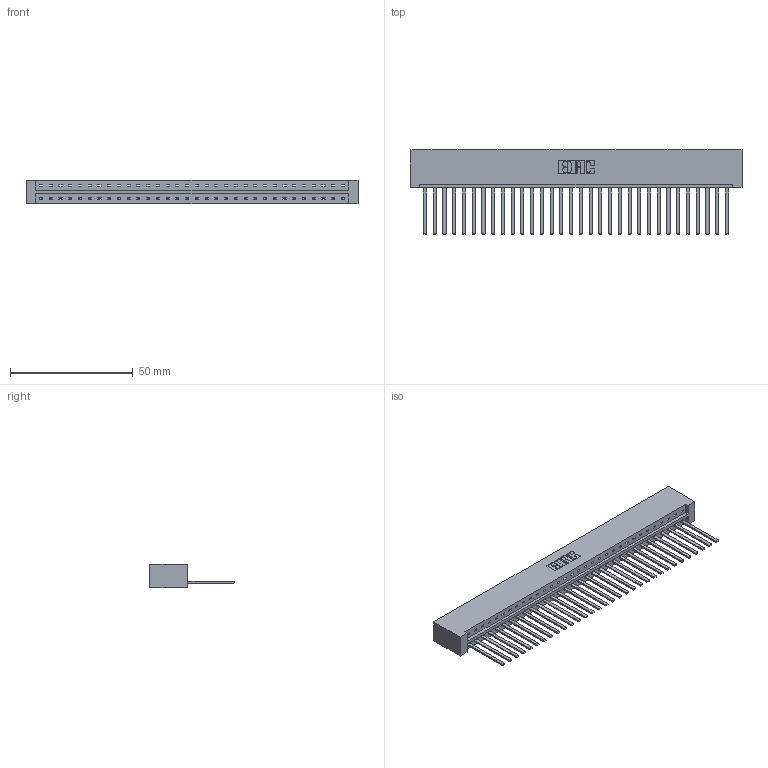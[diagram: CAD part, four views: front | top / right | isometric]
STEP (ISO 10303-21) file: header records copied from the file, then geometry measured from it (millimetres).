
FILE_DESCRIPTION (( 'STEP AP203' ), '1' );
FILE_NAME ('333-032-544-101.STEP', '2018-08-02T20:25:11', ( '' ), ( '' ), 'SwSTEP 2.0', 'SolidWorks 2016', '' );
FILE_SCHEMA (( 'CONFIG_CONTROL_DESIGN' ));
Length unit declared in the file: inch
Products named in the file (3): 333 Part_Lugless; 345-292-001_345-293-144; 333-032-544-101
Assembly tree (33 placements, depth 2):
  333-032-544-101
    333 Part_Lugless
    345-292-001_345-293-144  x32
Bounding box: 135.05 x 34.3 x 9.4 mm (x, y, z)
Volume: 14487.4 mm3; surface area: 16771.2 mm2
Topology: 33 solids, 33 shells, 1770 faces, 5343 edges, 3518 vertices
Faces by surface type: plane 1282, cylinder 488
Entity records: 20395 total; most frequent: CARTESIAN_POINT 3526, ORIENTED_EDGE 3494, DIRECTION 2983, EDGE_CURVE 1747, VECTOR 1631, LINE 1631, VERTEX_POINT 1162, AXIS2_PLACEMENT_3D 676
